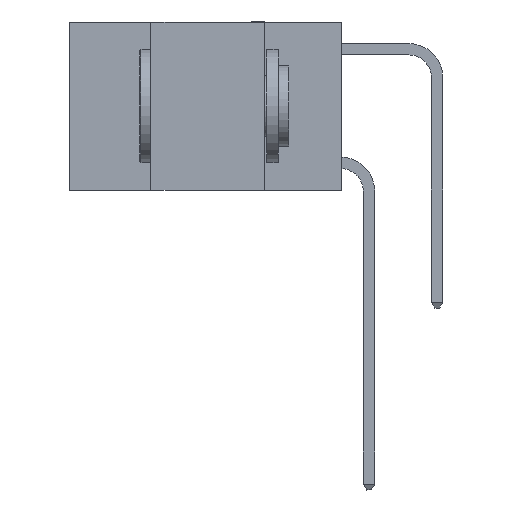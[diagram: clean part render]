
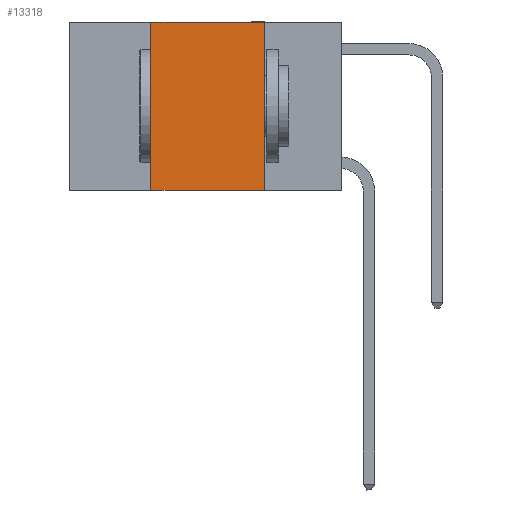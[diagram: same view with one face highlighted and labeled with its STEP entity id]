
A CAD part, left-side view. The second image highlights one B-rep face of the part: STEP entity #13318.
In plain terms, the highlighted planar face has unit normal (-1, 0, 0).
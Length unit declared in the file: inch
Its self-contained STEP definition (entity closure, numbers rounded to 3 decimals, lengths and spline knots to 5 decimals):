
#689 = VECTOR ( 'NONE', #15218, 39.37008 ) ;
#1036 = VECTOR ( 'NONE', #2371, 39.37008 ) ;
#1171 = LINE ( 'NONE', #6888, #689 ) ;
#1267 = VERTEX_POINT ( 'NONE', #15012 ) ;
#2242 = CARTESIAN_POINT ( 'NONE',  ( 0., 0.42, 0. ) ) ;
#2293 = CARTESIAN_POINT ( 'NONE',  ( 0., 0.17, 0. ) ) ;
#2371 = DIRECTION ( 'NONE',  ( 0., -1., 0. ) ) ;
#3376 = PLANE ( 'NONE',  #7305 ) ;
#3485 = CARTESIAN_POINT ( 'NONE',  ( 0., 0.6, 0. ) ) ;
#3633 = ORIENTED_EDGE ( 'NONE', *, *, #14512, .T. ) ;
#4037 = VERTEX_POINT ( 'NONE', #2293 ) ;
#4798 = FACE_OUTER_BOUND ( 'NONE', #7146, .T. ) ;
#4992 = VERTEX_POINT ( 'NONE', #9285 ) ;
#6490 = LINE ( 'NONE', #2242, #10702 ) ;
#6888 = CARTESIAN_POINT ( 'NONE',  ( 0., 0.6, 0. ) ) ;
#6896 = ORIENTED_EDGE ( 'NONE', *, *, #16301, .F. ) ;
#7146 = EDGE_LOOP ( 'NONE', ( #15897, #12299, #6896, #3633 ) ) ;
#7305 = AXIS2_PLACEMENT_3D ( 'NONE', #3485, #17725, #16131 ) ;
#9142 = CARTESIAN_POINT ( 'NONE',  ( 0., 0.42, 0. ) ) ;
#9277 = DIRECTION ( 'NONE',  ( 0., 0., 1. ) ) ;
#9285 = CARTESIAN_POINT ( 'NONE',  ( 0., 0.17, -0.37 ) ) ;
#9725 = VERTEX_POINT ( 'NONE', #9142 ) ;
#10702 = VECTOR ( 'NONE', #9277, 39.37008 ) ;
#10724 = LINE ( 'NONE', #16529, #1036 ) ;
#11160 = VECTOR ( 'NONE', #18036, 39.37008 ) ;
#11360 = EDGE_CURVE ( 'NONE', #9725, #4037, #1171, .T. ) ;
#12299 = ORIENTED_EDGE ( 'NONE', *, *, #11360, .F. ) ;
#12601 = LINE ( 'NONE', #18326, #11160 ) ;
#13318 = ADVANCED_FACE ( 'NONE', ( #4798 ), #3376, .F. ) ;
#14512 = EDGE_CURVE ( 'NONE', #1267, #4992, #10724, .T. ) ;
#15012 = CARTESIAN_POINT ( 'NONE',  ( 0., 0.42, -0.37 ) ) ;
#15218 = DIRECTION ( 'NONE',  ( 0., -1., 0. ) ) ;
#15897 = ORIENTED_EDGE ( 'NONE', *, *, #16889, .F. ) ;
#16131 = DIRECTION ( 'NONE',  ( 0., 0., -1. ) ) ;
#16301 = EDGE_CURVE ( 'NONE', #1267, #9725, #6490, .T. ) ;
#16529 = CARTESIAN_POINT ( 'NONE',  ( 0., 0.6, -0.37 ) ) ;
#16889 = EDGE_CURVE ( 'NONE', #4037, #4992, #12601, .T. ) ;
#17725 = DIRECTION ( 'NONE',  ( 1., 0., 0. ) ) ;
#18036 = DIRECTION ( 'NONE',  ( 0., 0., -1. ) ) ;
#18326 = CARTESIAN_POINT ( 'NONE',  ( 0., 0.17, 0. ) ) ;
